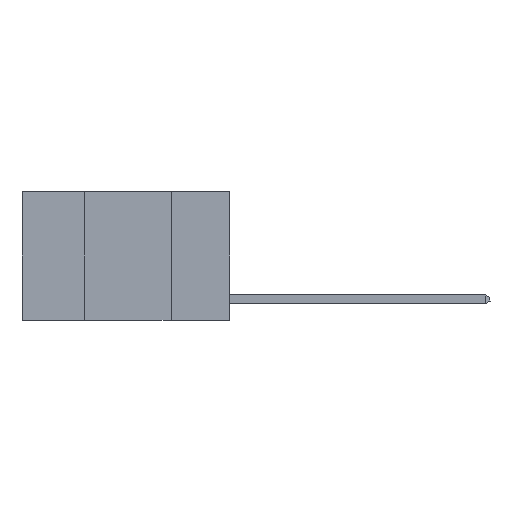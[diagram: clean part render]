
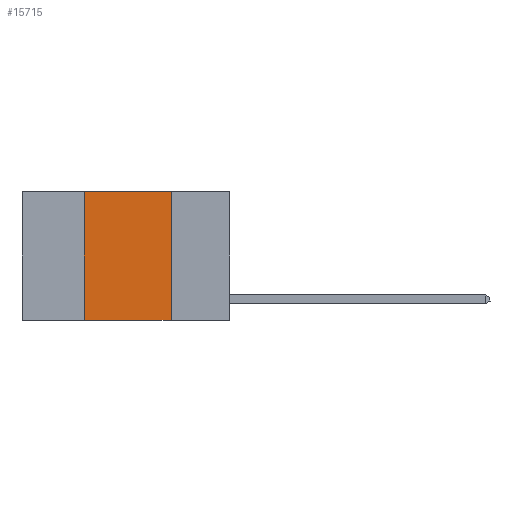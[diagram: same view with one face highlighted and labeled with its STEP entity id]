
A CAD part, left-side view. The second image highlights one B-rep face of the part: STEP entity #15715.
In plain terms, the highlighted planar face has unit normal (-1, 0, 0).
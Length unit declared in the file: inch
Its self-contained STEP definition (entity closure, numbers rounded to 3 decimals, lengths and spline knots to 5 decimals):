
#337 = VERTEX_POINT ( 'NONE', #5976 ) ;
#495 = CARTESIAN_POINT ( 'NONE',  ( 0., 0.17, 0. ) ) ;
#3226 = EDGE_CURVE ( 'NONE', #22847, #11130, #12606, .T. ) ;
#3250 = PLANE ( 'NONE',  #9964 ) ;
#3888 = LINE ( 'NONE', #18352, #23321 ) ;
#4102 = ORIENTED_EDGE ( 'NONE', *, *, #4238, .F. ) ;
#4238 = EDGE_CURVE ( 'NONE', #337, #22847, #17232, .T. ) ;
#4431 = EDGE_CURVE ( 'NONE', #8695, #337, #5201, .T. ) ;
#5201 = LINE ( 'NONE', #23741, #5467 ) ;
#5264 = VECTOR ( 'NONE', #15642, 39.37008 ) ;
#5467 = VECTOR ( 'NONE', #23887, 39.37008 ) ;
#5976 = CARTESIAN_POINT ( 'NONE',  ( 0., 0.42, 0. ) ) ;
#6191 = CARTESIAN_POINT ( 'NONE',  ( 0., 0.6, 0. ) ) ;
#7590 = CARTESIAN_POINT ( 'NONE',  ( 0., 0.17, -0.37 ) ) ;
#8695 = VERTEX_POINT ( 'NONE', #21159 ) ;
#9964 = AXIS2_PLACEMENT_3D ( 'NONE', #14589, #21553, #24008 ) ;
#11130 = VERTEX_POINT ( 'NONE', #7590 ) ;
#11232 = ORIENTED_EDGE ( 'NONE', *, *, #12830, .T. ) ;
#12469 = FACE_OUTER_BOUND ( 'NONE', #20163, .T. ) ;
#12606 = LINE ( 'NONE', #495, #5264 ) ;
#12830 = EDGE_CURVE ( 'NONE', #8695, #11130, #3888, .T. ) ;
#13115 = ORIENTED_EDGE ( 'NONE', *, *, #3226, .F. ) ;
#14589 = CARTESIAN_POINT ( 'NONE',  ( 0., 0.6, 0. ) ) ;
#15642 = DIRECTION ( 'NONE',  ( 0., 0., -1. ) ) ;
#15715 = ADVANCED_FACE ( 'NONE', ( #12469 ), #3250, .F. ) ;
#16957 = VECTOR ( 'NONE', #23086, 39.37008 ) ;
#17232 = LINE ( 'NONE', #6191, #16957 ) ;
#17566 = CARTESIAN_POINT ( 'NONE',  ( 0., 0.17, 0. ) ) ;
#18352 = CARTESIAN_POINT ( 'NONE',  ( 0., 0.6, -0.37 ) ) ;
#20163 = EDGE_LOOP ( 'NONE', ( #13115, #4102, #24250, #11232 ) ) ;
#21159 = CARTESIAN_POINT ( 'NONE',  ( 0., 0.42, -0.37 ) ) ;
#21553 = DIRECTION ( 'NONE',  ( 1., 0., 0. ) ) ;
#22847 = VERTEX_POINT ( 'NONE', #17566 ) ;
#23086 = DIRECTION ( 'NONE',  ( 0., -1., 0. ) ) ;
#23321 = VECTOR ( 'NONE', #23923, 39.37008 ) ;
#23741 = CARTESIAN_POINT ( 'NONE',  ( 0., 0.42, 0. ) ) ;
#23887 = DIRECTION ( 'NONE',  ( 0., 0., 1. ) ) ;
#23923 = DIRECTION ( 'NONE',  ( 0., -1., 0. ) ) ;
#24008 = DIRECTION ( 'NONE',  ( 0., 0., -1. ) ) ;
#24250 = ORIENTED_EDGE ( 'NONE', *, *, #4431, .F. ) ;
